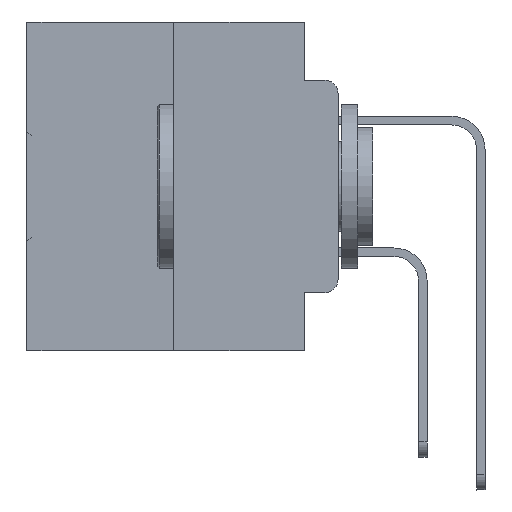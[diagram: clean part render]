
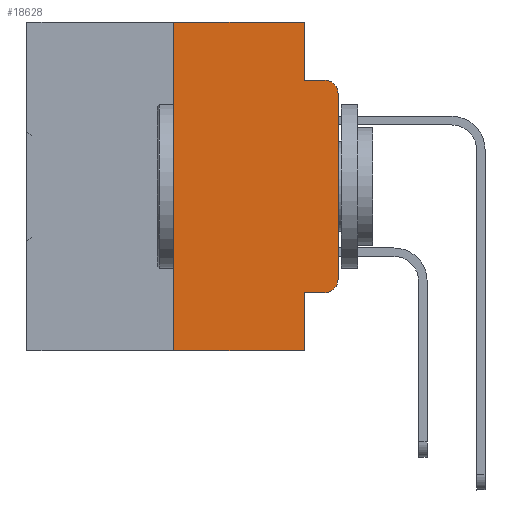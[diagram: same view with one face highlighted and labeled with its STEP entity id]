
A CAD part, left-side view. The second image highlights one B-rep face of the part: STEP entity #18628.
In plain terms, the highlighted planar face has unit normal (-1, 0, 0).
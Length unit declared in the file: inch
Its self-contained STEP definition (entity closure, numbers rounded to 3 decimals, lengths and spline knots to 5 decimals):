
#1158 = LINE ( 'NONE', #1940, #7820 ) ;
#1255 = LINE ( 'NONE', #16565, #7925 ) ;
#1369 = DIRECTION ( 'NONE',  ( 0., -1., 0. ) ) ;
#1467 = VERTEX_POINT ( 'NONE', #10145 ) ;
#1940 = CARTESIAN_POINT ( 'NONE',  ( 0., 0.051, 0. ) ) ;
#2360 = CARTESIAN_POINT ( 'NONE',  ( 0., 0.051, -0.0885 ) ) ;
#2453 = VERTEX_POINT ( 'NONE', #27330 ) ;
#2559 = CARTESIAN_POINT ( 'NONE',  ( 0., 0.051, -0.4115 ) ) ;
#2697 = AXIS2_PLACEMENT_3D ( 'NONE', #11651, #22714, #6039 ) ;
#3913 = ORIENTED_EDGE ( 'NONE', *, *, #24710, .T. ) ;
#4265 = EDGE_CURVE ( 'NONE', #8977, #2453, #20148, .T. ) ;
#4368 = ORIENTED_EDGE ( 'NONE', *, *, #4265, .F. ) ;
#4398 = VECTOR ( 'NONE', #7975, 39.37008 ) ;
#5537 = CARTESIAN_POINT ( 'NONE',  ( 0., 0., -0.1085 ) ) ;
#5803 = VERTEX_POINT ( 'NONE', #5537 ) ;
#6039 = DIRECTION ( 'NONE',  ( 0., 0., -1. ) ) ;
#7295 = VERTEX_POINT ( 'NONE', #12051 ) ;
#7643 = CARTESIAN_POINT ( 'NONE',  ( 0., 0.02, -0.1085 ) ) ;
#7766 = CARTESIAN_POINT ( 'NONE',  ( 0., 0., 0. ) ) ;
#7820 = VECTOR ( 'NONE', #15980, 39.37008 ) ;
#7925 = VECTOR ( 'NONE', #30079, 39.37008 ) ;
#7975 = DIRECTION ( 'NONE',  ( 0., 0., 1. ) ) ;
#8110 = VECTOR ( 'NONE', #16379, 39.37008 ) ;
#8438 = LINE ( 'NONE', #7766, #23164 ) ;
#8589 = CARTESIAN_POINT ( 'NONE',  ( 0., 0.25, 0. ) ) ;
#8767 = EDGE_CURVE ( 'NONE', #1467, #7295, #30334, .T. ) ;
#8977 = VERTEX_POINT ( 'NONE', #14668 ) ;
#10131 = ORIENTED_EDGE ( 'NONE', *, *, #11874, .F. ) ;
#10145 = CARTESIAN_POINT ( 'NONE',  ( 0., 0.02, -0.4115 ) ) ;
#10511 = DIRECTION ( 'NONE',  ( 0., 0., -1. ) ) ;
#10658 = CARTESIAN_POINT ( 'NONE',  ( 0., 0.051, -0.4115 ) ) ;
#11132 = CARTESIAN_POINT ( 'NONE',  ( 0., 0.02, -0.3915 ) ) ;
#11651 = CARTESIAN_POINT ( 'NONE',  ( 0., 0.473, 0. ) ) ;
#11775 = DIRECTION ( 'NONE',  ( 0., -1., 0. ) ) ;
#11874 = EDGE_CURVE ( 'NONE', #20657, #18231, #1158, .T. ) ;
#11913 = ORIENTED_EDGE ( 'NONE', *, *, #31492, .T. ) ;
#12051 = CARTESIAN_POINT ( 'NONE',  ( 0., 0., -0.3915 ) ) ;
#13162 = VERTEX_POINT ( 'NONE', #10658 ) ;
#13710 = EDGE_LOOP ( 'NONE', ( #3913, #20520, #31034, #10131, #25609, #4368, #11913, #20968, #29806, #16234 ) ) ;
#13718 = EDGE_CURVE ( 'NONE', #18231, #30287, #29985, .T. ) ;
#13933 = DIRECTION ( 'NONE',  ( 0., 0., -1. ) ) ;
#14668 = CARTESIAN_POINT ( 'NONE',  ( 0., 0.25, -0.5 ) ) ;
#15259 = EDGE_CURVE ( 'NONE', #2453, #20657, #15492, .T. ) ;
#15492 = LINE ( 'NONE', #34301, #16355 ) ;
#15980 = DIRECTION ( 'NONE',  ( 0., 0., -1. ) ) ;
#16234 = ORIENTED_EDGE ( 'NONE', *, *, #8767, .T. ) ;
#16254 = EDGE_CURVE ( 'NONE', #13162, #1467, #21031, .T. ) ;
#16355 = VECTOR ( 'NONE', #1369, 39.37008 ) ;
#16379 = DIRECTION ( 'NONE',  ( 0., -1., 0. ) ) ;
#16565 = CARTESIAN_POINT ( 'NONE',  ( 0., 0.051, 0. ) ) ;
#16770 = AXIS2_PLACEMENT_3D ( 'NONE', #11132, #30193, #13933 ) ;
#18231 = VERTEX_POINT ( 'NONE', #18429 ) ;
#18293 = LINE ( 'NONE', #33451, #32584 ) ;
#18429 = CARTESIAN_POINT ( 'NONE',  ( 0., 0.051, -0.0885 ) ) ;
#18628 = ADVANCED_FACE ( 'NONE', ( #33808 ), #30672, .F. ) ;
#19060 = CARTESIAN_POINT ( 'NONE',  ( 0., 0.051, 0. ) ) ;
#20148 = LINE ( 'NONE', #8589, #4398 ) ;
#20520 = ORIENTED_EDGE ( 'NONE', *, *, #22931, .T. ) ;
#20657 = VERTEX_POINT ( 'NONE', #19060 ) ;
#20968 = ORIENTED_EDGE ( 'NONE', *, *, #25399, .F. ) ;
#21031 = LINE ( 'NONE', #2559, #33577 ) ;
#22103 = DIRECTION ( 'NONE',  ( 0., -1., 0. ) ) ;
#22172 = CARTESIAN_POINT ( 'NONE',  ( 0., 0.02, -0.0885 ) ) ;
#22714 = DIRECTION ( 'NONE',  ( 1., 0., 0. ) ) ;
#22931 = EDGE_CURVE ( 'NONE', #5803, #30287, #30781, .T. ) ;
#23164 = VECTOR ( 'NONE', #27084, 39.37008 ) ;
#24710 = EDGE_CURVE ( 'NONE', #7295, #5803, #8438, .T. ) ;
#25399 = EDGE_CURVE ( 'NONE', #13162, #34566, #1255, .T. ) ;
#25609 = ORIENTED_EDGE ( 'NONE', *, *, #15259, .F. ) ;
#26960 = DIRECTION ( 'NONE',  ( -1., 0., 0. ) ) ;
#27084 = DIRECTION ( 'NONE',  ( 0., 0., 1. ) ) ;
#27330 = CARTESIAN_POINT ( 'NONE',  ( 0., 0.25, 0. ) ) ;
#29806 = ORIENTED_EDGE ( 'NONE', *, *, #16254, .T. ) ;
#29985 = LINE ( 'NONE', #2360, #8110 ) ;
#30010 = CARTESIAN_POINT ( 'NONE',  ( 0., 0.051, -0.5 ) ) ;
#30079 = DIRECTION ( 'NONE',  ( 0., 0., -1. ) ) ;
#30193 = DIRECTION ( 'NONE',  ( -1., 0., 0. ) ) ;
#30287 = VERTEX_POINT ( 'NONE', #22172 ) ;
#30334 = CIRCLE ( 'NONE', #16770, 0.02 ) ;
#30672 = PLANE ( 'NONE',  #2697 ) ;
#30781 = CIRCLE ( 'NONE', #32328, 0.02 ) ;
#31034 = ORIENTED_EDGE ( 'NONE', *, *, #13718, .F. ) ;
#31492 = EDGE_CURVE ( 'NONE', #8977, #34566, #18293, .T. ) ;
#32328 = AXIS2_PLACEMENT_3D ( 'NONE', #7643, #26960, #10511 ) ;
#32584 = VECTOR ( 'NONE', #11775, 39.37008 ) ;
#33451 = CARTESIAN_POINT ( 'NONE',  ( 0., 0.473, -0.5 ) ) ;
#33577 = VECTOR ( 'NONE', #22103, 39.37008 ) ;
#33808 = FACE_OUTER_BOUND ( 'NONE', #13710, .T. ) ;
#34301 = CARTESIAN_POINT ( 'NONE',  ( 0., 0.473, 0. ) ) ;
#34566 = VERTEX_POINT ( 'NONE', #30010 ) ;
